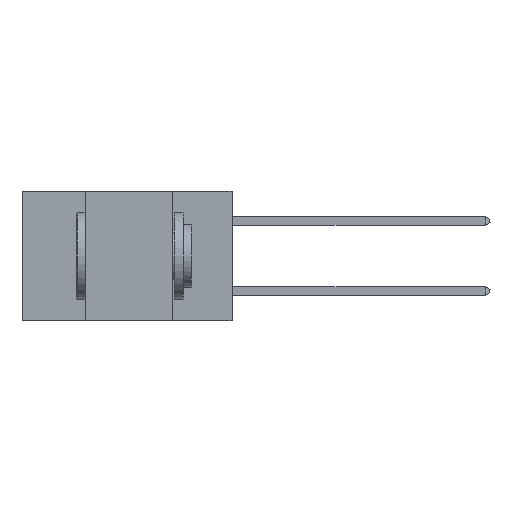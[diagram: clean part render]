
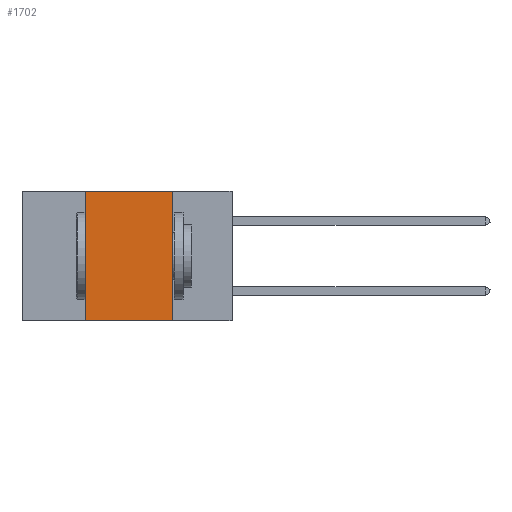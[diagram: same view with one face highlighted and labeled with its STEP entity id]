
A CAD part, left-side view. The second image highlights one B-rep face of the part: STEP entity #1702.
In plain terms, the highlighted planar face has unit normal (-1, 0, 0).
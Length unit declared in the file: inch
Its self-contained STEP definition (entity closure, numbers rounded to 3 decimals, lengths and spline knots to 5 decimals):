
#462 = VECTOR ( 'NONE', #11969, 39.37008 ) ;
#591 = CARTESIAN_POINT ( 'NONE',  ( 0., 0.6, 0. ) ) ;
#998 = CARTESIAN_POINT ( 'NONE',  ( 0., 0.17, -0.37 ) ) ;
#1391 = DIRECTION ( 'NONE',  ( 0., 0., -1. ) ) ;
#1536 = CARTESIAN_POINT ( 'NONE',  ( 0., 0.42, 0. ) ) ;
#1702 = ADVANCED_FACE ( 'NONE', ( #37051 ), #30252, .F. ) ;
#3618 = LINE ( 'NONE', #19390, #35283 ) ;
#7120 = EDGE_CURVE ( 'NONE', #14712, #14920, #12795, .T. ) ;
#8686 = CARTESIAN_POINT ( 'NONE',  ( 0., 0.42, -0.37 ) ) ;
#11245 = ORIENTED_EDGE ( 'NONE', *, *, #27486, .F. ) ;
#11936 = EDGE_CURVE ( 'NONE', #13789, #14712, #23622, .T. ) ;
#11969 = DIRECTION ( 'NONE',  ( 0., 0., 1. ) ) ;
#12795 = LINE ( 'NONE', #591, #27579 ) ;
#13033 = DIRECTION ( 'NONE',  ( 1., 0., 0. ) ) ;
#13789 = VERTEX_POINT ( 'NONE', #8686 ) ;
#14712 = VERTEX_POINT ( 'NONE', #1536 ) ;
#14920 = VERTEX_POINT ( 'NONE', #25200 ) ;
#17538 = CARTESIAN_POINT ( 'NONE',  ( 0., 0.42, 0. ) ) ;
#17728 = ORIENTED_EDGE ( 'NONE', *, *, #17769, .T. ) ;
#17769 = EDGE_CURVE ( 'NONE', #13789, #34086, #33889, .T. ) ;
#18527 = VECTOR ( 'NONE', #21547, 39.37008 ) ;
#18737 = CARTESIAN_POINT ( 'NONE',  ( 0., 0.6, 0. ) ) ;
#19390 = CARTESIAN_POINT ( 'NONE',  ( 0., 0.17, 0. ) ) ;
#21547 = DIRECTION ( 'NONE',  ( 0., -1., 0. ) ) ;
#23622 = LINE ( 'NONE', #17538, #462 ) ;
#24465 = CARTESIAN_POINT ( 'NONE',  ( 0., 0.6, -0.37 ) ) ;
#25200 = CARTESIAN_POINT ( 'NONE',  ( 0., 0.17, 0. ) ) ;
#27486 = EDGE_CURVE ( 'NONE', #14920, #34086, #3618, .T. ) ;
#27579 = VECTOR ( 'NONE', #29588, 39.37008 ) ;
#28822 = DIRECTION ( 'NONE',  ( 0., 0., -1. ) ) ;
#29588 = DIRECTION ( 'NONE',  ( 0., -1., 0. ) ) ;
#29610 = EDGE_LOOP ( 'NONE', ( #11245, #32834, #31410, #17728 ) ) ;
#30252 = PLANE ( 'NONE',  #34119 ) ;
#31410 = ORIENTED_EDGE ( 'NONE', *, *, #11936, .F. ) ;
#32834 = ORIENTED_EDGE ( 'NONE', *, *, #7120, .F. ) ;
#33889 = LINE ( 'NONE', #24465, #18527 ) ;
#34086 = VERTEX_POINT ( 'NONE', #998 ) ;
#34119 = AXIS2_PLACEMENT_3D ( 'NONE', #18737, #13033, #1391 ) ;
#35283 = VECTOR ( 'NONE', #28822, 39.37008 ) ;
#37051 = FACE_OUTER_BOUND ( 'NONE', #29610, .T. ) ;
